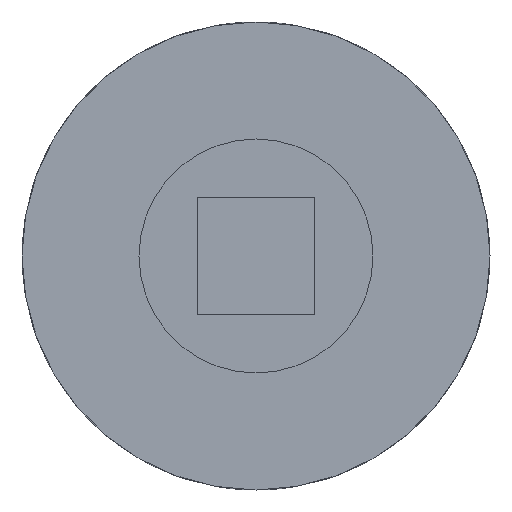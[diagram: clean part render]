
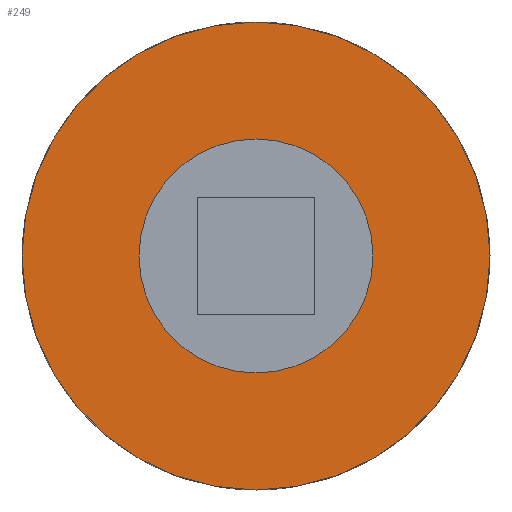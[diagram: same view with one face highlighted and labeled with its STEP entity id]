
A CAD part, front view. The second image highlights one B-rep face of the part: STEP entity #249.
In plain terms, the highlighted planar face has unit normal (0, -1, 0).
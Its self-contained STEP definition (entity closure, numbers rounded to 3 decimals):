
#7 = AXIS2_PLACEMENT_3D ( 'NONE', #26, #715, #219 ) ;
#23 = FACE_OUTER_BOUND ( 'NONE', #93, .T. ) ;
#26 = CARTESIAN_POINT ( 'NONE',  ( 0., 0., 0. ) ) ;
#54 = AXIS2_PLACEMENT_3D ( 'NONE', #631, #800, #946 ) ;
#93 = EDGE_LOOP ( 'NONE', ( #173, #237 ) ) ;
#121 = EDGE_LOOP ( 'NONE', ( #153, #170 ) ) ;
#147 = EDGE_CURVE ( 'NONE', #493, #547, #931, .T. ) ;
#153 = ORIENTED_EDGE ( 'NONE', *, *, #903, .T. ) ;
#170 = ORIENTED_EDGE ( 'NONE', *, *, #474, .T. ) ;
#173 = ORIENTED_EDGE ( 'NONE', *, *, #147, .F. ) ;
#186 = DIRECTION ( 'NONE',  ( 0., 0., 1. ) ) ;
#196 = DIRECTION ( 'NONE',  ( 0., 0., 1. ) ) ;
#219 = DIRECTION ( 'NONE',  ( 0., 0., 1. ) ) ;
#237 = ORIENTED_EDGE ( 'NONE', *, *, #641, .F. ) ;
#249 = ADVANCED_FACE ( 'NONE', ( #797, #23 ), #254, .F. ) ;
#254 = PLANE ( 'NONE',  #7 ) ;
#260 = DIRECTION ( 'NONE',  ( 0., 1., 0. ) ) ;
#262 = CARTESIAN_POINT ( 'NONE',  ( 0., 0., 0. ) ) ;
#312 = CARTESIAN_POINT ( 'NONE',  ( 0., 0., 0. ) ) ;
#361 = CIRCLE ( 'NONE', #810, 10. ) ;
#474 = EDGE_CURVE ( 'NONE', #570, #696, #361, .T. ) ;
#493 = VERTEX_POINT ( 'NONE', #520 ) ;
#520 = CARTESIAN_POINT ( 'NONE',  ( 0., 0., -20. ) ) ;
#522 = CIRCLE ( 'NONE', #688, 10. ) ;
#547 = VERTEX_POINT ( 'NONE', #922 ) ;
#552 = DIRECTION ( 'NONE',  ( 0., 0., 1. ) ) ;
#570 = VERTEX_POINT ( 'NONE', #773 ) ;
#597 = CIRCLE ( 'NONE', #710, 20. ) ;
#631 = CARTESIAN_POINT ( 'NONE',  ( 0., 0., 0. ) ) ;
#641 = EDGE_CURVE ( 'NONE', #547, #493, #597, .T. ) ;
#688 = AXIS2_PLACEMENT_3D ( 'NONE', #791, #708, #552 ) ;
#696 = VERTEX_POINT ( 'NONE', #904 ) ;
#708 = DIRECTION ( 'NONE',  ( 0., 1., 0. ) ) ;
#709 = DIRECTION ( 'NONE',  ( 0., 1., 0. ) ) ;
#710 = AXIS2_PLACEMENT_3D ( 'NONE', #312, #709, #196 ) ;
#715 = DIRECTION ( 'NONE',  ( 0., 1., 0. ) ) ;
#773 = CARTESIAN_POINT ( 'NONE',  ( 0., 0., -10. ) ) ;
#791 = CARTESIAN_POINT ( 'NONE',  ( 0., 0., 0. ) ) ;
#797 = FACE_BOUND ( 'NONE', #121, .T. ) ;
#800 = DIRECTION ( 'NONE',  ( 0., 1., 0. ) ) ;
#810 = AXIS2_PLACEMENT_3D ( 'NONE', #262, #260, #186 ) ;
#903 = EDGE_CURVE ( 'NONE', #696, #570, #522, .T. ) ;
#904 = CARTESIAN_POINT ( 'NONE',  ( 0., 0., 10. ) ) ;
#922 = CARTESIAN_POINT ( 'NONE',  ( 0., 0., 20. ) ) ;
#931 = CIRCLE ( 'NONE', #54, 20. ) ;
#946 = DIRECTION ( 'NONE',  ( 0., 0., 1. ) ) ;
